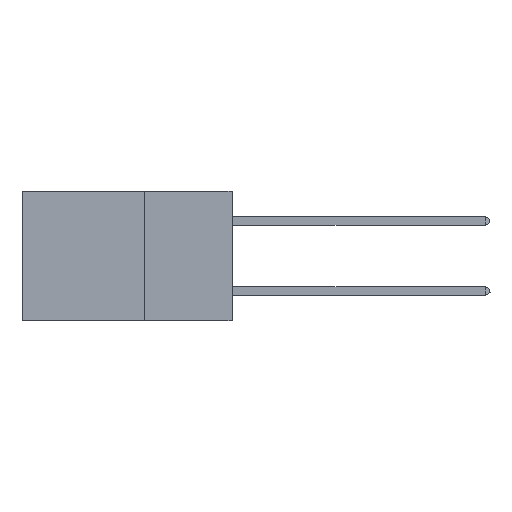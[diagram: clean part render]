
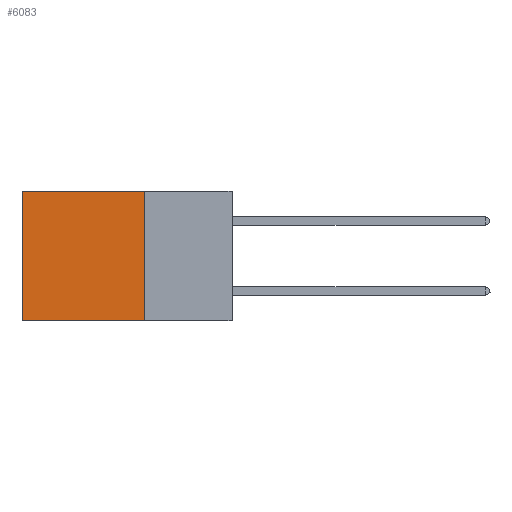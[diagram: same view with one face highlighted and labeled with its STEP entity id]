
A CAD part, left-side view. The second image highlights one B-rep face of the part: STEP entity #6083.
In plain terms, the highlighted planar face has unit normal (-1, 0, 0).
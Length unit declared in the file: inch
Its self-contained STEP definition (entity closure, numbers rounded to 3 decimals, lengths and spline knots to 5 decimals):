
#3 = DIRECTION ( 'NONE',  ( 0., 1., 0. ) ) ;
#2240 = CARTESIAN_POINT ( 'NONE',  ( 0.2875, 0.25, 0. ) ) ;
#2839 = LINE ( 'NONE', #2240, #23428 ) ;
#2886 = EDGE_LOOP ( 'NONE', ( #9613, #11771, #20668, #13332 ) ) ;
#5715 = VECTOR ( 'NONE', #3, 39.37008 ) ;
#6083 = ADVANCED_FACE ( 'NONE', ( #8393 ), #8006, .F. ) ;
#7531 = CARTESIAN_POINT ( 'NONE',  ( 0.2875, 0.25, -0.37 ) ) ;
#8006 = PLANE ( 'NONE',  #16826 ) ;
#8083 = DIRECTION ( 'NONE',  ( 0., 1., 0. ) ) ;
#8393 = FACE_OUTER_BOUND ( 'NONE', #2886, .T. ) ;
#9198 = VERTEX_POINT ( 'NONE', #30385 ) ;
#9453 = VERTEX_POINT ( 'NONE', #9693 ) ;
#9613 = ORIENTED_EDGE ( 'NONE', *, *, #30546, .T. ) ;
#9693 = CARTESIAN_POINT ( 'NONE',  ( 0.2875, 0.25, -0.37 ) ) ;
#11771 = ORIENTED_EDGE ( 'NONE', *, *, #30118, .F. ) ;
#12519 = LINE ( 'NONE', #7531, #5715 ) ;
#13332 = ORIENTED_EDGE ( 'NONE', *, *, #21112, .T. ) ;
#16826 = AXIS2_PLACEMENT_3D ( 'NONE', #21804, #24561, #19613 ) ;
#16898 = LINE ( 'NONE', #24674, #29471 ) ;
#17775 = VECTOR ( 'NONE', #8083, 39.37008 ) ;
#19387 = DIRECTION ( 'NONE',  ( 0., 0., -1. ) ) ;
#19613 = DIRECTION ( 'NONE',  ( 0., 0., -1. ) ) ;
#20668 = ORIENTED_EDGE ( 'NONE', *, *, #26481, .F. ) ;
#20941 = LINE ( 'NONE', #30614, #17775 ) ;
#21112 = EDGE_CURVE ( 'NONE', #9198, #22097, #20941, .T. ) ;
#21804 = CARTESIAN_POINT ( 'NONE',  ( 0.2875, 0.25, 0. ) ) ;
#21966 = CARTESIAN_POINT ( 'NONE',  ( 0.2875, 0.6, 0. ) ) ;
#22097 = VERTEX_POINT ( 'NONE', #21966 ) ;
#23428 = VECTOR ( 'NONE', #27663, 39.37008 ) ;
#23938 = VERTEX_POINT ( 'NONE', #31992 ) ;
#24561 = DIRECTION ( 'NONE',  ( 1., 0., 0. ) ) ;
#24674 = CARTESIAN_POINT ( 'NONE',  ( 0.2875, 0.6, 0. ) ) ;
#26481 = EDGE_CURVE ( 'NONE', #9198, #9453, #2839, .T. ) ;
#27663 = DIRECTION ( 'NONE',  ( 0., 0., -1. ) ) ;
#29471 = VECTOR ( 'NONE', #19387, 39.37008 ) ;
#30118 = EDGE_CURVE ( 'NONE', #9453, #23938, #12519, .T. ) ;
#30385 = CARTESIAN_POINT ( 'NONE',  ( 0.2875, 0.25, 0. ) ) ;
#30546 = EDGE_CURVE ( 'NONE', #22097, #23938, #16898, .T. ) ;
#30614 = CARTESIAN_POINT ( 'NONE',  ( 0.2875, 0.25, 0. ) ) ;
#31992 = CARTESIAN_POINT ( 'NONE',  ( 0.2875, 0.6, -0.37 ) ) ;
